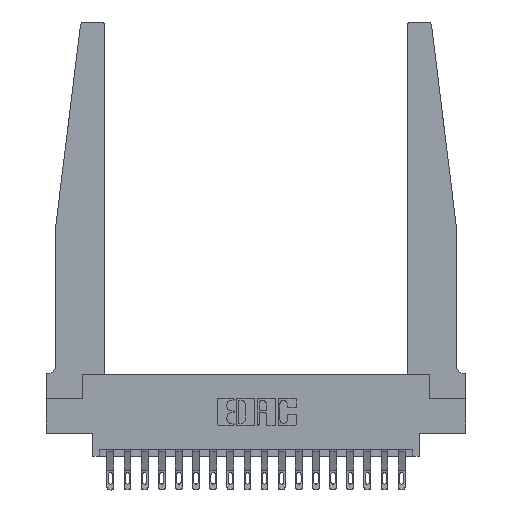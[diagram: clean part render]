
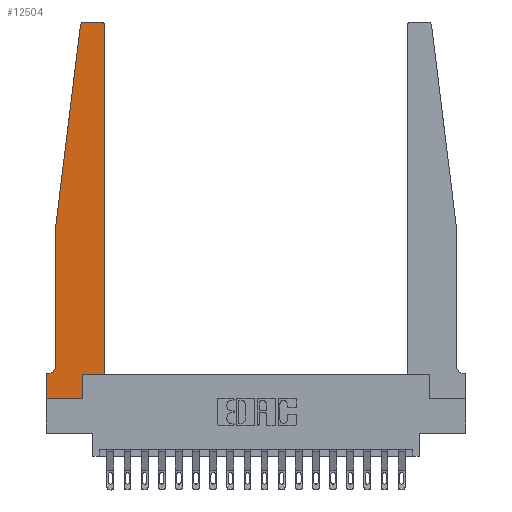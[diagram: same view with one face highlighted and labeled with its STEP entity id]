
A CAD part, top view. The second image highlights one B-rep face of the part: STEP entity #12504.
In plain terms, the highlighted planar face has unit normal (0, 0, 1).
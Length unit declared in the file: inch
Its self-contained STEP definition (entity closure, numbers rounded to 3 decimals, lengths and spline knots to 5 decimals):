
#9 = VERTEX_POINT ( 'NONE', #1677 ) ;
#269 = ORIENTED_EDGE ( 'NONE', *, *, #18608, .T. ) ;
#676 = CARTESIAN_POINT ( 'NONE',  ( 0.25, 2.75, 0.37 ) ) ;
#872 = CIRCLE ( 'NONE', #15393, 0.03 ) ;
#898 = CARTESIAN_POINT ( 'NONE',  ( 0.2605, 0.18, 0.37 ) ) ;
#913 = PLANE ( 'NONE',  #6027 ) ;
#1018 = DIRECTION ( 'NONE',  ( 1., 0., 0. ) ) ;
#1211 = ORIENTED_EDGE ( 'NONE', *, *, #3384, .T. ) ;
#1517 = DIRECTION ( 'NONE',  ( -1., 0., 0. ) ) ;
#1619 = DIRECTION ( 'NONE',  ( 0., 0., 1. ) ) ;
#1677 = CARTESIAN_POINT ( 'NONE',  ( 0.065, 1.25, 0.37 ) ) ;
#1912 = LINE ( 'NONE', #5904, #13899 ) ;
#2382 = EDGE_CURVE ( 'NONE', #4283, #5158, #6117, .T. ) ;
#2509 = DIRECTION ( 'NONE',  ( 1., 0., 0. ) ) ;
#2520 = VECTOR ( 'NONE', #5435, 39.37008 ) ;
#2541 = LINE ( 'NONE', #8654, #10402 ) ;
#2926 = ORIENTED_EDGE ( 'NONE', *, *, #10125, .T. ) ;
#2944 = VECTOR ( 'NONE', #12353, 39.37008 ) ;
#3073 = VERTEX_POINT ( 'NONE', #9908 ) ;
#3127 = ORIENTED_EDGE ( 'NONE', *, *, #7783, .T. ) ;
#3227 = ORIENTED_EDGE ( 'NONE', *, *, #6585, .T. ) ;
#3324 = ORIENTED_EDGE ( 'NONE', *, *, #7247, .T. ) ;
#3384 = EDGE_CURVE ( 'NONE', #9, #5335, #1912, .T. ) ;
#3412 = EDGE_CURVE ( 'NONE', #5821, #11067, #5597, .T. ) ;
#3497 = DIRECTION ( 'NONE',  ( 0., 0., 1. ) ) ;
#4040 = ORIENTED_EDGE ( 'NONE', *, *, #3412, .T. ) ;
#4239 = VECTOR ( 'NONE', #13279, 39.37008 ) ;
#4283 = VERTEX_POINT ( 'NONE', #19398 ) ;
#4895 = VERTEX_POINT ( 'NONE', #18068 ) ;
#5158 = VERTEX_POINT ( 'NONE', #18733 ) ;
#5335 = VERTEX_POINT ( 'NONE', #8352 ) ;
#5435 = DIRECTION ( 'NONE',  ( -1., 0., 0. ) ) ;
#5593 = CARTESIAN_POINT ( 'NONE',  ( 0., 0.1875, 0.37 ) ) ;
#5597 = LINE ( 'NONE', #13751, #17987 ) ;
#5821 = VERTEX_POINT ( 'NONE', #15601 ) ;
#5845 = AXIS2_PLACEMENT_3D ( 'NONE', #12845, #3497, #14395 ) ;
#5904 = CARTESIAN_POINT ( 'NONE',  ( 0.065, 1.25, 0.37 ) ) ;
#6027 = AXIS2_PLACEMENT_3D ( 'NONE', #5593, #11878, #2509 ) ;
#6117 = CIRCLE ( 'NONE', #5845, 0.03 ) ;
#6585 = EDGE_CURVE ( 'NONE', #5158, #9, #18108, .T. ) ;
#6630 = VERTEX_POINT ( 'NONE', #17866 ) ;
#6690 = ORIENTED_EDGE ( 'NONE', *, *, #16323, .T. ) ;
#6732 = EDGE_CURVE ( 'NONE', #19529, #5821, #6937, .T. ) ;
#6937 = LINE ( 'NONE', #898, #4239 ) ;
#7247 = EDGE_CURVE ( 'NONE', #4895, #15010, #2541, .T. ) ;
#7290 = CARTESIAN_POINT ( 'NONE',  ( 0.015, 0.1875, 0.37 ) ) ;
#7783 = EDGE_CURVE ( 'NONE', #6630, #4283, #15439, .T. ) ;
#8352 = CARTESIAN_POINT ( 'NONE',  ( 0.065, 0.2375, 0.37 ) ) ;
#8441 = CARTESIAN_POINT ( 'NONE',  ( 0.065, 1.25, 0.37 ) ) ;
#8654 = CARTESIAN_POINT ( 'NONE',  ( 0., 0., 0.37 ) ) ;
#8842 = CARTESIAN_POINT ( 'NONE',  ( 0., 0., 0.37 ) ) ;
#8923 = CARTESIAN_POINT ( 'NONE',  ( 0., 0., 0.37 ) ) ;
#8932 = ORIENTED_EDGE ( 'NONE', *, *, #20179, .T. ) ;
#9588 = ORIENTED_EDGE ( 'NONE', *, *, #2382, .T. ) ;
#9908 = CARTESIAN_POINT ( 'NONE',  ( 0.425, 2.72, 0.37 ) ) ;
#10125 = EDGE_CURVE ( 'NONE', #3073, #6630, #872, .T. ) ;
#10182 = DIRECTION ( 'NONE',  ( -1., 0., 0. ) ) ;
#10272 = DIRECTION ( 'NONE',  ( 0., -1., 0. ) ) ;
#10402 = VECTOR ( 'NONE', #10272, 39.37008 ) ;
#10656 = CIRCLE ( 'NONE', #19496, 0.05 ) ;
#10802 = CARTESIAN_POINT ( 'NONE',  ( 0.425, 0.18, 0.37 ) ) ;
#10932 = DIRECTION ( 'NONE',  ( 0., 0., -1. ) ) ;
#11032 = CARTESIAN_POINT ( 'NONE',  ( 0.395, 2.72, 0.37 ) ) ;
#11067 = VERTEX_POINT ( 'NONE', #13426 ) ;
#11181 = EDGE_LOOP ( 'NONE', ( #3127, #9588, #3227, #1211, #6690, #269, #3324, #13603, #13338, #4040, #8932, #2926 ) ) ;
#11800 = VECTOR ( 'NONE', #10182, 39.37008 ) ;
#11878 = DIRECTION ( 'NONE',  ( 0., 0., 1. ) ) ;
#12285 = LINE ( 'NONE', #19444, #11800 ) ;
#12353 = DIRECTION ( 'NONE',  ( 0., 1., 0. ) ) ;
#12504 = ADVANCED_FACE ( 'NONE', ( #14230 ), #913, .T. ) ;
#12581 = DIRECTION ( 'NONE',  ( 1., 0., 0. ) ) ;
#12845 = CARTESIAN_POINT ( 'NONE',  ( 0.27653, 2.72, 0.37 ) ) ;
#12999 = LINE ( 'NONE', #8842, #16598 ) ;
#13148 = DIRECTION ( 'NONE',  ( -0.122, -0.992, 0. ) ) ;
#13197 = VERTEX_POINT ( 'NONE', #7290 ) ;
#13198 = EDGE_CURVE ( 'NONE', #15010, #19529, #12999, .T. ) ;
#13279 = DIRECTION ( 'NONE',  ( 0., 1., 0. ) ) ;
#13338 = ORIENTED_EDGE ( 'NONE', *, *, #6732, .T. ) ;
#13426 = CARTESIAN_POINT ( 'NONE',  ( 0.425, 0.18, 0.37 ) ) ;
#13603 = ORIENTED_EDGE ( 'NONE', *, *, #13198, .T. ) ;
#13751 = CARTESIAN_POINT ( 'NONE',  ( 0.425, 0.18, 0.37 ) ) ;
#13899 = VECTOR ( 'NONE', #16770, 39.37008 ) ;
#14230 = FACE_OUTER_BOUND ( 'NONE', #11181, .T. ) ;
#14395 = DIRECTION ( 'NONE',  ( 1., 0., 0. ) ) ;
#14397 = LINE ( 'NONE', #10802, #2944 ) ;
#15010 = VERTEX_POINT ( 'NONE', #8923 ) ;
#15298 = DIRECTION ( 'NONE',  ( 1., 0., 0. ) ) ;
#15393 = AXIS2_PLACEMENT_3D ( 'NONE', #11032, #1619, #12581 ) ;
#15439 = LINE ( 'NONE', #676, #2520 ) ;
#15601 = CARTESIAN_POINT ( 'NONE',  ( 0.2605, 0.18, 0.37 ) ) ;
#16323 = EDGE_CURVE ( 'NONE', #5335, #13197, #10656, .T. ) ;
#16598 = VECTOR ( 'NONE', #1018, 39.37008 ) ;
#16770 = DIRECTION ( 'NONE',  ( 0., -1., 0. ) ) ;
#17128 = VECTOR ( 'NONE', #13148, 39.37008 ) ;
#17866 = CARTESIAN_POINT ( 'NONE',  ( 0.395, 2.75, 0.37 ) ) ;
#17987 = VECTOR ( 'NONE', #15298, 39.37008 ) ;
#18068 = CARTESIAN_POINT ( 'NONE',  ( 0., 0.1875, 0.37 ) ) ;
#18108 = LINE ( 'NONE', #8441, #17128 ) ;
#18608 = EDGE_CURVE ( 'NONE', #13197, #4895, #12285, .T. ) ;
#18733 = CARTESIAN_POINT ( 'NONE',  ( 0.24675, 2.72367, 0.37 ) ) ;
#19398 = CARTESIAN_POINT ( 'NONE',  ( 0.27653, 2.75, 0.37 ) ) ;
#19444 = CARTESIAN_POINT ( 'NONE',  ( 0.065, 0.1875, 0.37 ) ) ;
#19496 = AXIS2_PLACEMENT_3D ( 'NONE', #20193, #10932, #1517 ) ;
#19529 = VERTEX_POINT ( 'NONE', #20085 ) ;
#20085 = CARTESIAN_POINT ( 'NONE',  ( 0.2605, 0., 0.37 ) ) ;
#20179 = EDGE_CURVE ( 'NONE', #11067, #3073, #14397, .T. ) ;
#20193 = CARTESIAN_POINT ( 'NONE',  ( 0.015, 0.2375, 0.37 ) ) ;
